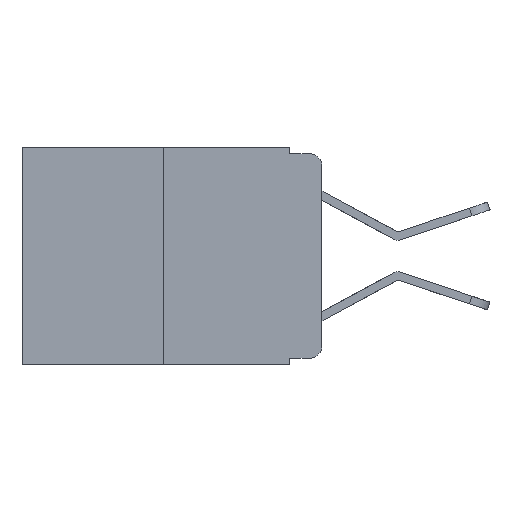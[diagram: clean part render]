
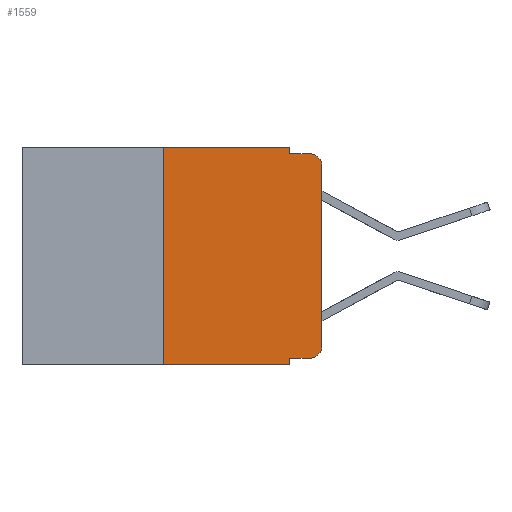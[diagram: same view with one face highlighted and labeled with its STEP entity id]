
A CAD part, left-side view. The second image highlights one B-rep face of the part: STEP entity #1559.
In plain terms, the highlighted planar face has unit normal (-1, 0, 0).
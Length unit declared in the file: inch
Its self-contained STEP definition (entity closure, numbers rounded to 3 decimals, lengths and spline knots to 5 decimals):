
#172 = DIRECTION ( 'NONE',  ( 0., 0., -1. ) ) ;
#340 = CARTESIAN_POINT ( 'NONE',  ( 0., 0.051, 0. ) ) ;
#424 = CARTESIAN_POINT ( 'NONE',  ( 0., 0.473, -0.343 ) ) ;
#942 = CARTESIAN_POINT ( 'NONE',  ( 0., 0.25, -0.343 ) ) ;
#1005 = CARTESIAN_POINT ( 'NONE',  ( 0., 0.051, -0.343 ) ) ;
#1127 = CARTESIAN_POINT ( 'NONE',  ( 0., 0.473, 0. ) ) ;
#1559 = ADVANCED_FACE ( 'NONE', ( #3768 ), #7175, .F. ) ;
#1840 = VECTOR ( 'NONE', #21474, 39.37008 ) ;
#1881 = ORIENTED_EDGE ( 'NONE', *, *, #13773, .T. ) ;
#1910 = EDGE_CURVE ( 'NONE', #3818, #2569, #21733, .T. ) ;
#2147 = CARTESIAN_POINT ( 'NONE',  ( 0., 0.02, -0.03 ) ) ;
#2569 = VERTEX_POINT ( 'NONE', #19198 ) ;
#3282 = EDGE_CURVE ( 'NONE', #11642, #15435, #7177, .T. ) ;
#3768 = FACE_OUTER_BOUND ( 'NONE', #18807, .T. ) ;
#3789 = ORIENTED_EDGE ( 'NONE', *, *, #1910, .T. ) ;
#3818 = VERTEX_POINT ( 'NONE', #19205 ) ;
#3935 = VERTEX_POINT ( 'NONE', #18770 ) ;
#4593 = VERTEX_POINT ( 'NONE', #942 ) ;
#4881 = CARTESIAN_POINT ( 'NONE',  ( 0., 0.02, -0.333 ) ) ;
#5051 = DIRECTION ( 'NONE',  ( 0., -1., 0. ) ) ;
#5207 = CARTESIAN_POINT ( 'NONE',  ( 0., 0.051, -0.01 ) ) ;
#5279 = EDGE_CURVE ( 'NONE', #20703, #2569, #21060, .T. ) ;
#5355 = DIRECTION ( 'NONE',  ( 1., 0., 0. ) ) ;
#5467 = EDGE_CURVE ( 'NONE', #9993, #17704, #19791, .T. ) ;
#5504 = EDGE_CURVE ( 'NONE', #4593, #3935, #9252, .T. ) ;
#5909 = DIRECTION ( 'NONE',  ( 0., -1., 0. ) ) ;
#6042 = ORIENTED_EDGE ( 'NONE', *, *, #23579, .T. ) ;
#6189 = ORIENTED_EDGE ( 'NONE', *, *, #5279, .F. ) ;
#6767 = DIRECTION ( 'NONE',  ( 0., 0., -1. ) ) ;
#7148 = VECTOR ( 'NONE', #18215, 39.37008 ) ;
#7175 = PLANE ( 'NONE',  #16521 ) ;
#7177 = LINE ( 'NONE', #340, #16456 ) ;
#7292 = VECTOR ( 'NONE', #17990, 39.37008 ) ;
#7686 = DIRECTION ( 'NONE',  ( 0., 0., -1. ) ) ;
#7828 = VECTOR ( 'NONE', #6767, 39.37008 ) ;
#7856 = CARTESIAN_POINT ( 'NONE',  ( 0., 0.25, 0. ) ) ;
#8498 = VERTEX_POINT ( 'NONE', #13152 ) ;
#8611 = ORIENTED_EDGE ( 'NONE', *, *, #9815, .T. ) ;
#8621 = CARTESIAN_POINT ( 'NONE',  ( 0., 0., 0. ) ) ;
#9252 = LINE ( 'NONE', #7856, #1840 ) ;
#9462 = ORIENTED_EDGE ( 'NONE', *, *, #3282, .F. ) ;
#9564 = ORIENTED_EDGE ( 'NONE', *, *, #15209, .F. ) ;
#9705 = LINE ( 'NONE', #20985, #7828 ) ;
#9815 = EDGE_CURVE ( 'NONE', #17704, #3818, #19261, .T. ) ;
#9932 = DIRECTION ( 'NONE',  ( -1., 0., 0. ) ) ;
#9993 = VERTEX_POINT ( 'NONE', #4881 ) ;
#10716 = CARTESIAN_POINT ( 'NONE',  ( 0., 0.473, 0. ) ) ;
#11065 = EDGE_CURVE ( 'NONE', #3935, #8498, #24753, .T. ) ;
#11642 = VERTEX_POINT ( 'NONE', #24209 ) ;
#11726 = CARTESIAN_POINT ( 'NONE',  ( 0., 0., -0.313 ) ) ;
#11968 = CARTESIAN_POINT ( 'NONE',  ( 0., 0.051, -0.01 ) ) ;
#12034 = VECTOR ( 'NONE', #5909, 39.37008 ) ;
#13139 = DIRECTION ( 'NONE',  ( 0., 0., -1. ) ) ;
#13152 = CARTESIAN_POINT ( 'NONE',  ( 0., 0.051, 0. ) ) ;
#13773 = EDGE_CURVE ( 'NONE', #4593, #15435, #17814, .T. ) ;
#15209 = EDGE_CURVE ( 'NONE', #8498, #20703, #9705, .T. ) ;
#15435 = VERTEX_POINT ( 'NONE', #1005 ) ;
#15491 = DIRECTION ( 'NONE',  ( -1., 0., 0. ) ) ;
#16048 = VECTOR ( 'NONE', #5051, 39.37008 ) ;
#16456 = VECTOR ( 'NONE', #172, 39.37008 ) ;
#16521 = AXIS2_PLACEMENT_3D ( 'NONE', #1127, #5355, #13139 ) ;
#17322 = LINE ( 'NONE', #20404, #16048 ) ;
#17704 = VERTEX_POINT ( 'NONE', #11726 ) ;
#17814 = LINE ( 'NONE', #424, #7292 ) ;
#17969 = VECTOR ( 'NONE', #22346, 39.37008 ) ;
#17990 = DIRECTION ( 'NONE',  ( 0., -1., 0. ) ) ;
#18215 = DIRECTION ( 'NONE',  ( 0., 0., 1. ) ) ;
#18770 = CARTESIAN_POINT ( 'NONE',  ( 0., 0.25, 0. ) ) ;
#18807 = EDGE_LOOP ( 'NONE', ( #8611, #3789, #6189, #9564, #22610, #20708, #1881, #9462, #6042, #25508 ) ) ;
#19198 = CARTESIAN_POINT ( 'NONE',  ( 0., 0.02, -0.01 ) ) ;
#19205 = CARTESIAN_POINT ( 'NONE',  ( 0., 0., -0.03 ) ) ;
#19261 = LINE ( 'NONE', #8621, #7148 ) ;
#19791 = CIRCLE ( 'NONE', #24364, 0.02 ) ;
#20404 = CARTESIAN_POINT ( 'NONE',  ( 0., 0.051, -0.333 ) ) ;
#20703 = VERTEX_POINT ( 'NONE', #5207 ) ;
#20708 = ORIENTED_EDGE ( 'NONE', *, *, #5504, .F. ) ;
#20985 = CARTESIAN_POINT ( 'NONE',  ( 0., 0.051, 0. ) ) ;
#21060 = LINE ( 'NONE', #11968, #12034 ) ;
#21474 = DIRECTION ( 'NONE',  ( 0., 0., 1. ) ) ;
#21733 = CIRCLE ( 'NONE', #24989, 0.02 ) ;
#22346 = DIRECTION ( 'NONE',  ( 0., -1., 0. ) ) ;
#22610 = ORIENTED_EDGE ( 'NONE', *, *, #11065, .F. ) ;
#23579 = EDGE_CURVE ( 'NONE', #11642, #9993, #17322, .T. ) ;
#23626 = CARTESIAN_POINT ( 'NONE',  ( 0., 0.02, -0.313 ) ) ;
#23795 = DIRECTION ( 'NONE',  ( 0., 0., -1. ) ) ;
#24209 = CARTESIAN_POINT ( 'NONE',  ( 0., 0.051, -0.333 ) ) ;
#24364 = AXIS2_PLACEMENT_3D ( 'NONE', #23626, #15491, #7686 ) ;
#24753 = LINE ( 'NONE', #10716, #17969 ) ;
#24989 = AXIS2_PLACEMENT_3D ( 'NONE', #2147, #9932, #23795 ) ;
#25508 = ORIENTED_EDGE ( 'NONE', *, *, #5467, .T. ) ;
